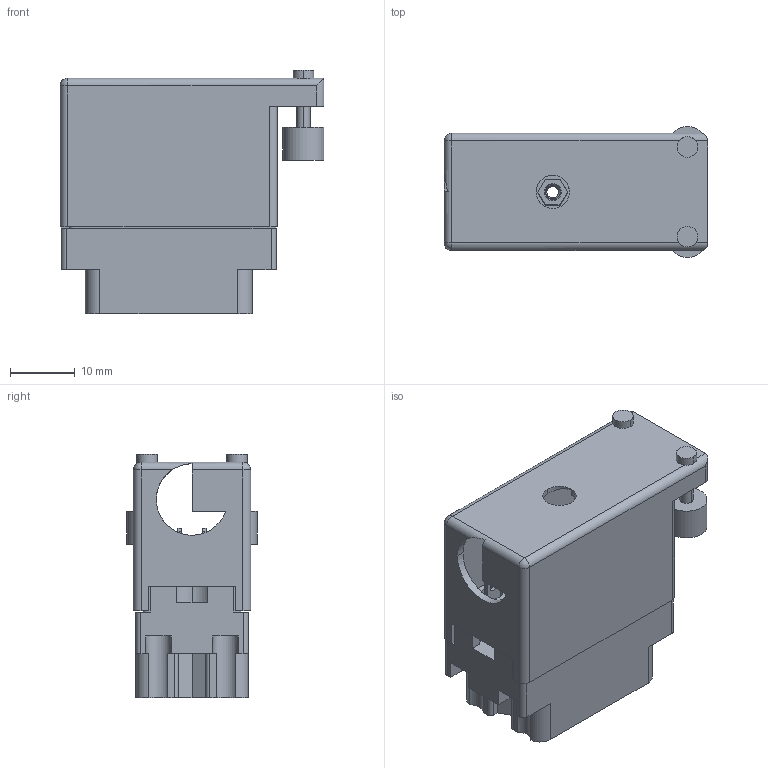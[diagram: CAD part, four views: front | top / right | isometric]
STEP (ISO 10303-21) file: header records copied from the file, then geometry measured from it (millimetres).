
FILE_DESCRIPTION (( 'STEP AP203' ), '1' );
FILE_NAME ('516-020-500-126.STEP', '2020-03-09T13:46:40', ( '' ), ( '' ), 'SwSTEP 2.0', 'SolidWorks 2016', '' );
FILE_SCHEMA (( 'CONFIG_CONTROL_DESIGN' ));
Length unit declared in the file: inch
Products named in the file (5): 516-020-500-126; 516-292-001_500 Contact; 516 Plug Insulator_020; 516-230-001_Plastic - 020 Side Entry; 516-252-025-100_516-252-025-100
Assembly tree (23 placements, depth 2):
  516-020-500-126
    516 Plug Insulator_020
    516-292-001_500 Contact  x20
    516-230-001_Plastic - 020 Side Entry
    516-252-025-100_516-252-025-100
Bounding box: 40.87 x 20.24 x 37.77 mm (x, y, z)
Volume: 8917.1 mm3; surface area: 16954.6 mm2
Topology: 23 solids, 23 shells, 2255 faces, 6545 edges, 4340 vertices
Faces by surface type: plane 1337, cylinder 782, bspline 123, cone 11, sphere 2
Entity records: 30852 total; most frequent: CARTESIAN_POINT 7832, ORIENTED_EDGE 4726, DIRECTION 4511, EDGE_CURVE 2363, LINE 1673, VECTOR 1673, VERTEX_POINT 1566, AXIS2_PLACEMENT_3D 1419
